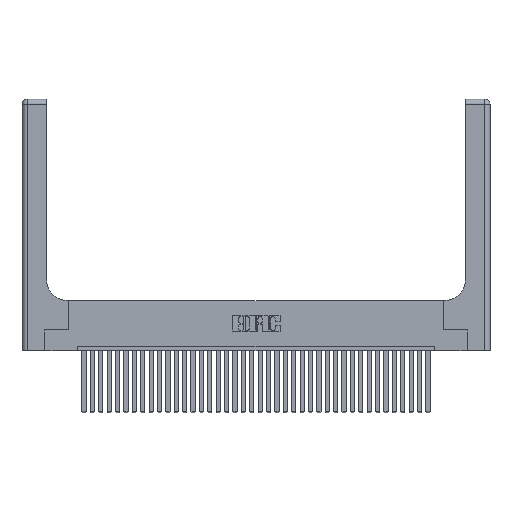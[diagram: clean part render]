
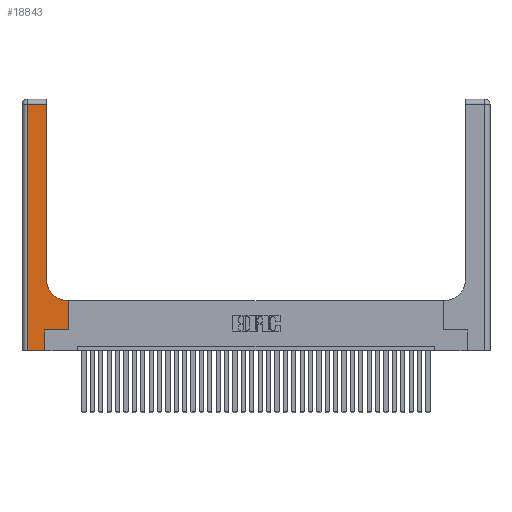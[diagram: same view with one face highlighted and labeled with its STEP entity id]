
A CAD part, top view. The second image highlights one B-rep face of the part: STEP entity #18843.
In plain terms, the highlighted planar face has unit normal (0, 0, 1).
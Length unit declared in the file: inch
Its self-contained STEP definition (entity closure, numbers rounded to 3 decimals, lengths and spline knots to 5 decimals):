
#16 = VERTEX_POINT ( 'NONE', #22010 ) ;
#118 = VERTEX_POINT ( 'NONE', #16074 ) ;
#220 = EDGE_LOOP ( 'NONE', ( #6508, #1331, #35086, #22584, #7857, #16619, #15205, #35807, #20866 ) ) ;
#695 = VERTEX_POINT ( 'NONE', #14305 ) ;
#1004 = CARTESIAN_POINT ( 'NONE',  ( 0.5585, 0.6, 0.37 ) ) ;
#1331 = ORIENTED_EDGE ( 'NONE', *, *, #13524, .T. ) ;
#1878 = EDGE_CURVE ( 'NONE', #26986, #695, #7913, .T. ) ;
#1898 = CARTESIAN_POINT ( 'NONE',  ( 0.06, 0., 0.37 ) ) ;
#4167 = EDGE_CURVE ( 'NONE', #15107, #9261, #21801, .T. ) ;
#4183 = DIRECTION ( 'NONE',  ( -1., 0., 0. ) ) ;
#4219 = CARTESIAN_POINT ( 'NONE',  ( 0.269, 0.25, 0.37 ) ) ;
#5665 = DIRECTION ( 'NONE',  ( 0., -1., 0. ) ) ;
#5901 = VECTOR ( 'NONE', #19374, 39.37008 ) ;
#6311 = DIRECTION ( 'NONE',  ( 1., 0., 0. ) ) ;
#6379 = DIRECTION ( 'NONE',  ( 1., 0., 0. ) ) ;
#6508 = ORIENTED_EDGE ( 'NONE', *, *, #26597, .T. ) ;
#6774 = DIRECTION ( 'NONE',  ( 0., 1., 0. ) ) ;
#7401 = EDGE_CURVE ( 'NONE', #9261, #118, #26507, .T. ) ;
#7559 = VECTOR ( 'NONE', #6379, 39.37008 ) ;
#7568 = CARTESIAN_POINT ( 'NONE',  ( 0.2915, 2.94, 0.37 ) ) ;
#7857 = ORIENTED_EDGE ( 'NONE', *, *, #35382, .T. ) ;
#7913 = LINE ( 'NONE', #32046, #34423 ) ;
#8154 = VECTOR ( 'NONE', #21429, 39.37008 ) ;
#9261 = VERTEX_POINT ( 'NONE', #31899 ) ;
#11870 = CARTESIAN_POINT ( 'NONE',  ( 0.5585, 0.25, 0.37 ) ) ;
#12318 = AXIS2_PLACEMENT_3D ( 'NONE', #22962, #17656, #6311 ) ;
#13444 = DIRECTION ( 'NONE',  ( 0., 1., 0. ) ) ;
#13524 = EDGE_CURVE ( 'NONE', #29260, #16, #35261, .T. ) ;
#13621 = EDGE_CURVE ( 'NONE', #24632, #15107, #20632, .T. ) ;
#13817 = CARTESIAN_POINT ( 'NONE',  ( 0.06, 3., 0.37 ) ) ;
#14305 = CARTESIAN_POINT ( 'NONE',  ( 0.269, 0., 0.37 ) ) ;
#15107 = VERTEX_POINT ( 'NONE', #1004 ) ;
#15205 = ORIENTED_EDGE ( 'NONE', *, *, #13621, .T. ) ;
#15264 = EDGE_CURVE ( 'NONE', #32812, #24632, #16823, .T. ) ;
#15645 = LINE ( 'NONE', #32426, #8154 ) ;
#16074 = CARTESIAN_POINT ( 'NONE',  ( 0.2915, 0.85, 0.37 ) ) ;
#16619 = ORIENTED_EDGE ( 'NONE', *, *, #15264, .T. ) ;
#16823 = LINE ( 'NONE', #29059, #7559 ) ;
#17122 = LINE ( 'NONE', #27502, #25066 ) ;
#17656 = DIRECTION ( 'NONE',  ( 0., 0., -1. ) ) ;
#17721 = CARTESIAN_POINT ( 'NONE',  ( 0., 2.94, 0.37 ) ) ;
#17818 = DIRECTION ( 'NONE',  ( 1., 0., 0. ) ) ;
#18106 = PLANE ( 'NONE',  #18401 ) ;
#18401 = AXIS2_PLACEMENT_3D ( 'NONE', #23775, #26267, #4183 ) ;
#18843 = ADVANCED_FACE ( 'NONE', ( #31642 ), #18106, .F. ) ;
#19374 = DIRECTION ( 'NONE',  ( -1., 0., 0. ) ) ;
#20324 = DIRECTION ( 'NONE',  ( -1., 0., 0. ) ) ;
#20632 = LINE ( 'NONE', #26275, #22815 ) ;
#20866 = ORIENTED_EDGE ( 'NONE', *, *, #7401, .T. ) ;
#21429 = DIRECTION ( 'NONE',  ( 0., 1., 0. ) ) ;
#21801 = LINE ( 'NONE', #24889, #5901 ) ;
#22010 = CARTESIAN_POINT ( 'NONE',  ( 0.06, 2.94, 0.37 ) ) ;
#22584 = ORIENTED_EDGE ( 'NONE', *, *, #1878, .T. ) ;
#22815 = VECTOR ( 'NONE', #6774, 39.37008 ) ;
#22962 = CARTESIAN_POINT ( 'NONE',  ( 0.5415, 0.85, 0.37 ) ) ;
#23775 = CARTESIAN_POINT ( 'NONE',  ( 0., 3., 0.37 ) ) ;
#24632 = VERTEX_POINT ( 'NONE', #11870 ) ;
#24889 = CARTESIAN_POINT ( 'NONE',  ( 0.2915, 0.6, 0.37 ) ) ;
#25066 = VECTOR ( 'NONE', #13444, 39.37008 ) ;
#25124 = LINE ( 'NONE', #13817, #26453 ) ;
#26267 = DIRECTION ( 'NONE',  ( 0., 0., -1. ) ) ;
#26275 = CARTESIAN_POINT ( 'NONE',  ( 0.5585, 0.25, 0.37 ) ) ;
#26453 = VECTOR ( 'NONE', #5665, 39.37008 ) ;
#26507 = CIRCLE ( 'NONE', #12318, 0.25 ) ;
#26597 = EDGE_CURVE ( 'NONE', #118, #29260, #15645, .T. ) ;
#26986 = VERTEX_POINT ( 'NONE', #1898 ) ;
#27502 = CARTESIAN_POINT ( 'NONE',  ( 0.269, 0., 0.37 ) ) ;
#29059 = CARTESIAN_POINT ( 'NONE',  ( 0.269, 0.25, 0.37 ) ) ;
#29260 = VERTEX_POINT ( 'NONE', #7568 ) ;
#31532 = EDGE_CURVE ( 'NONE', #16, #26986, #25124, .T. ) ;
#31642 = FACE_OUTER_BOUND ( 'NONE', #220, .T. ) ;
#31899 = CARTESIAN_POINT ( 'NONE',  ( 0.5415, 0.6, 0.37 ) ) ;
#32046 = CARTESIAN_POINT ( 'NONE',  ( 0., 0., 0.37 ) ) ;
#32426 = CARTESIAN_POINT ( 'NONE',  ( 0.2915, 3., 0.37 ) ) ;
#32812 = VERTEX_POINT ( 'NONE', #4219 ) ;
#34379 = VECTOR ( 'NONE', #20324, 39.37008 ) ;
#34423 = VECTOR ( 'NONE', #17818, 39.37008 ) ;
#35086 = ORIENTED_EDGE ( 'NONE', *, *, #31532, .T. ) ;
#35261 = LINE ( 'NONE', #17721, #34379 ) ;
#35382 = EDGE_CURVE ( 'NONE', #695, #32812, #17122, .T. ) ;
#35807 = ORIENTED_EDGE ( 'NONE', *, *, #4167, .T. ) ;
